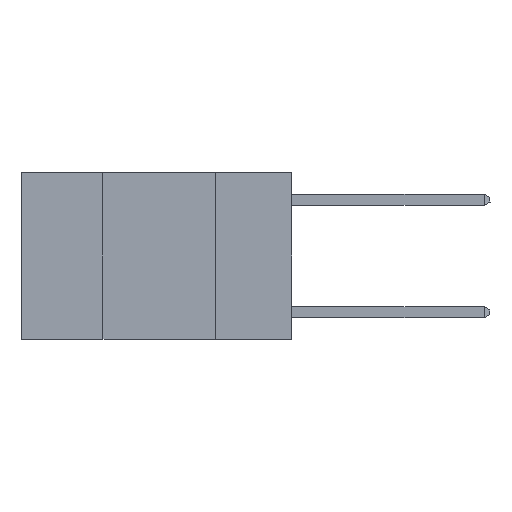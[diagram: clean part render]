
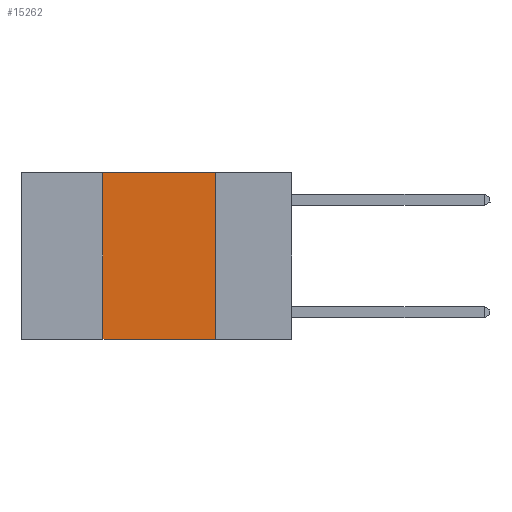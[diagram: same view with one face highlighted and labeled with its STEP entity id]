
A CAD part, left-side view. The second image highlights one B-rep face of the part: STEP entity #15262.
In plain terms, the highlighted planar face has unit normal (-1, 0, 0).
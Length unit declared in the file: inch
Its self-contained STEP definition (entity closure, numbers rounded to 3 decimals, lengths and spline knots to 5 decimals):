
#78 = EDGE_CURVE ( 'NONE', #933, #8442, #22711, .T. ) ;
#933 = VERTEX_POINT ( 'NONE', #4068 ) ;
#1468 = CARTESIAN_POINT ( 'NONE',  ( 0., 0.17, 0. ) ) ;
#2741 = EDGE_CURVE ( 'NONE', #18091, #20394, #10331, .T. ) ;
#4068 = CARTESIAN_POINT ( 'NONE',  ( 0., 0.42, -0.37 ) ) ;
#7937 = CARTESIAN_POINT ( 'NONE',  ( 0., 0.6, -0.37 ) ) ;
#8219 = CARTESIAN_POINT ( 'NONE',  ( 0., 0.6, 0. ) ) ;
#8442 = VERTEX_POINT ( 'NONE', #15874 ) ;
#8444 = LINE ( 'NONE', #12320, #24075 ) ;
#8828 = EDGE_CURVE ( 'NONE', #933, #18091, #14046, .T. ) ;
#8932 = ORIENTED_EDGE ( 'NONE', *, *, #23063, .F. ) ;
#9698 = ORIENTED_EDGE ( 'NONE', *, *, #2741, .F. ) ;
#9703 = ORIENTED_EDGE ( 'NONE', *, *, #8828, .F. ) ;
#9880 = EDGE_LOOP ( 'NONE', ( #8932, #9698, #9703, #10398 ) ) ;
#10331 = LINE ( 'NONE', #20774, #20966 ) ;
#10398 = ORIENTED_EDGE ( 'NONE', *, *, #78, .T. ) ;
#10401 = DIRECTION ( 'NONE',  ( 0., 0., -1. ) ) ;
#10777 = CARTESIAN_POINT ( 'NONE',  ( 0., 0.42, 0. ) ) ;
#11177 = FACE_OUTER_BOUND ( 'NONE', #9880, .T. ) ;
#12320 = CARTESIAN_POINT ( 'NONE',  ( 0., 0.17, 0. ) ) ;
#14046 = LINE ( 'NONE', #10777, #25986 ) ;
#14226 = AXIS2_PLACEMENT_3D ( 'NONE', #8219, #23087, #10401 ) ;
#14470 = DIRECTION ( 'NONE',  ( 0., 0., -1. ) ) ;
#15262 = ADVANCED_FACE ( 'NONE', ( #11177 ), #20986, .F. ) ;
#15874 = CARTESIAN_POINT ( 'NONE',  ( 0., 0.17, -0.37 ) ) ;
#18091 = VERTEX_POINT ( 'NONE', #22705 ) ;
#20394 = VERTEX_POINT ( 'NONE', #1468 ) ;
#20774 = CARTESIAN_POINT ( 'NONE',  ( 0., 0.6, 0. ) ) ;
#20966 = VECTOR ( 'NONE', #25042, 39.37008 ) ;
#20986 = PLANE ( 'NONE',  #14226 ) ;
#22060 = VECTOR ( 'NONE', #22808, 39.37008 ) ;
#22705 = CARTESIAN_POINT ( 'NONE',  ( 0., 0.42, 0. ) ) ;
#22711 = LINE ( 'NONE', #7937, #22060 ) ;
#22808 = DIRECTION ( 'NONE',  ( 0., -1., 0. ) ) ;
#23063 = EDGE_CURVE ( 'NONE', #20394, #8442, #8444, .T. ) ;
#23087 = DIRECTION ( 'NONE',  ( 1., 0., 0. ) ) ;
#24075 = VECTOR ( 'NONE', #14470, 39.37008 ) ;
#25042 = DIRECTION ( 'NONE',  ( 0., -1., 0. ) ) ;
#25646 = DIRECTION ( 'NONE',  ( 0., 0., 1. ) ) ;
#25986 = VECTOR ( 'NONE', #25646, 39.37008 ) ;
